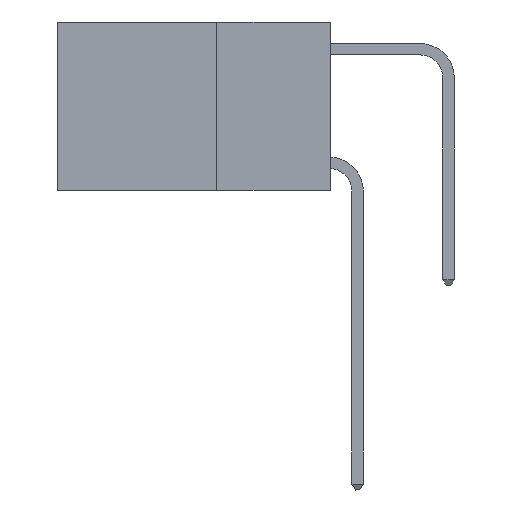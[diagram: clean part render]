
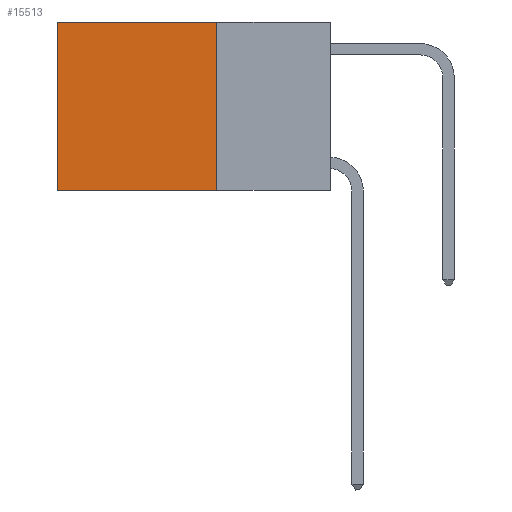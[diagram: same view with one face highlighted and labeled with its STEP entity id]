
A CAD part, left-side view. The second image highlights one B-rep face of the part: STEP entity #15513.
In plain terms, the highlighted planar face has unit normal (-1, 0, 0).
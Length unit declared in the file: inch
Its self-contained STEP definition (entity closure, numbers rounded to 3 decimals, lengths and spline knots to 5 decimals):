
#160 = CARTESIAN_POINT ( 'NONE',  ( 0.2625, 0.25, -0.37 ) ) ;
#197 = EDGE_CURVE ( 'NONE', #7661, #15339, #6511, .T. ) ;
#545 = CARTESIAN_POINT ( 'NONE',  ( 0.2625, 0.6, -0.37 ) ) ;
#1056 = DIRECTION ( 'NONE',  ( 0., 0., -1. ) ) ;
#1872 = VERTEX_POINT ( 'NONE', #4924 ) ;
#2079 = VECTOR ( 'NONE', #3047, 39.37008 ) ;
#2278 = LINE ( 'NONE', #13128, #2079 ) ;
#3047 = DIRECTION ( 'NONE',  ( 0., 0., -1. ) ) ;
#3154 = PLANE ( 'NONE',  #7259 ) ;
#3245 = EDGE_LOOP ( 'NONE', ( #13502, #15243, #14100, #4424 ) ) ;
#3414 = CARTESIAN_POINT ( 'NONE',  ( 0.2625, 0.25, 0. ) ) ;
#3514 = VECTOR ( 'NONE', #5230, 39.37008 ) ;
#3892 = CARTESIAN_POINT ( 'NONE',  ( 0.2625, 0.6, 0. ) ) ;
#4424 = ORIENTED_EDGE ( 'NONE', *, *, #197, .T. ) ;
#4924 = CARTESIAN_POINT ( 'NONE',  ( 0.2625, 0.25, -0.37 ) ) ;
#5230 = DIRECTION ( 'NONE',  ( 0., 1., 0. ) ) ;
#6511 = LINE ( 'NONE', #8581, #11051 ) ;
#6708 = EDGE_CURVE ( 'NONE', #1872, #15730, #10230, .T. ) ;
#6825 = EDGE_CURVE ( 'NONE', #15339, #15730, #2278, .T. ) ;
#7259 = AXIS2_PLACEMENT_3D ( 'NONE', #10787, #13277, #14580 ) ;
#7661 = VERTEX_POINT ( 'NONE', #3414 ) ;
#8581 = CARTESIAN_POINT ( 'NONE',  ( 0.2625, 0.25, 0. ) ) ;
#9338 = VECTOR ( 'NONE', #1056, 39.37008 ) ;
#9988 = CARTESIAN_POINT ( 'NONE',  ( 0.2625, 0.25, 0. ) ) ;
#10230 = LINE ( 'NONE', #160, #3514 ) ;
#10787 = CARTESIAN_POINT ( 'NONE',  ( 0.2625, 0.25, 0. ) ) ;
#11051 = VECTOR ( 'NONE', #12342, 39.37008 ) ;
#12117 = FACE_OUTER_BOUND ( 'NONE', #3245, .T. ) ;
#12342 = DIRECTION ( 'NONE',  ( 0., 1., 0. ) ) ;
#13128 = CARTESIAN_POINT ( 'NONE',  ( 0.2625, 0.6, 0. ) ) ;
#13277 = DIRECTION ( 'NONE',  ( 1., 0., 0. ) ) ;
#13502 = ORIENTED_EDGE ( 'NONE', *, *, #6825, .T. ) ;
#14100 = ORIENTED_EDGE ( 'NONE', *, *, #15694, .F. ) ;
#14580 = DIRECTION ( 'NONE',  ( 0., 0., -1. ) ) ;
#15243 = ORIENTED_EDGE ( 'NONE', *, *, #6708, .F. ) ;
#15339 = VERTEX_POINT ( 'NONE', #3892 ) ;
#15513 = ADVANCED_FACE ( 'NONE', ( #12117 ), #3154, .F. ) ;
#15694 = EDGE_CURVE ( 'NONE', #7661, #1872, #15883, .T. ) ;
#15730 = VERTEX_POINT ( 'NONE', #545 ) ;
#15883 = LINE ( 'NONE', #9988, #9338 ) ;
